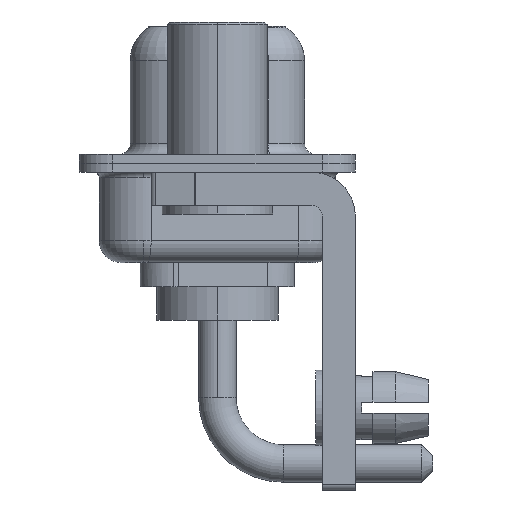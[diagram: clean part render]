
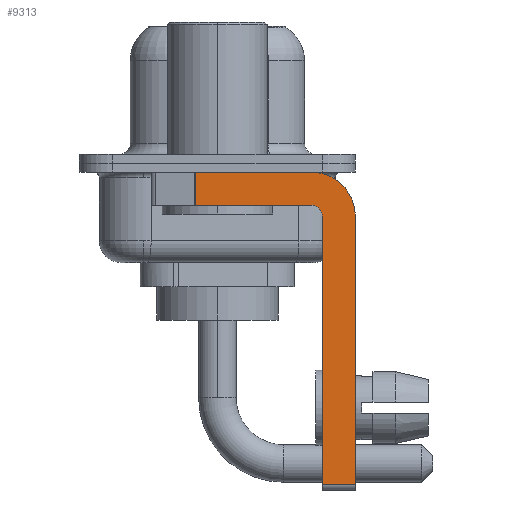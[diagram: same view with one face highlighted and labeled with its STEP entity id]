
A CAD part, left-side view. The second image highlights one B-rep face of the part: STEP entity #9313.
In plain terms, the highlighted planar face has unit normal (-1, 0, 0).
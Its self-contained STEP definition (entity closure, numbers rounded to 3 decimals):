
#875 = CARTESIAN_POINT ( 'NONE',  ( -2.9, -6.25, -14.55 ) ) ;
#929 = CARTESIAN_POINT ( 'NONE',  ( -2.9, -6.25, -2.4 ) ) ;
#1006 = DIRECTION ( 'NONE',  ( 0., -1., 0. ) ) ;
#1123 = EDGE_CURVE ( 'NONE', #10890, #2275, #14505, .T. ) ;
#1128 = VECTOR ( 'NONE', #12689, 1000. ) ;
#1149 = EDGE_CURVE ( 'NONE', #10330, #9300, #10543, .T. ) ;
#1270 = CIRCLE ( 'NONE', #10921, 0.5 ) ;
#1470 = EDGE_CURVE ( 'NONE', #8513, #6060, #1560, .T. ) ;
#1560 = CIRCLE ( 'NONE', #10450, 2. ) ;
#1697 = CARTESIAN_POINT ( 'NONE',  ( -2.9, -4.25, -2.4 ) ) ;
#1864 = DIRECTION ( 'NONE',  ( 0., 0., -1. ) ) ;
#2187 = CARTESIAN_POINT ( 'NONE',  ( -2.9, -4.25, -14.55 ) ) ;
#2262 = CARTESIAN_POINT ( 'NONE',  ( -2.9, -4.25, -2.4 ) ) ;
#2275 = VERTEX_POINT ( 'NONE', #7239 ) ;
#2492 = ORIENTED_EDGE ( 'NONE', *, *, #4163, .T. ) ;
#2978 = VERTEX_POINT ( 'NONE', #14285 ) ;
#2998 = CARTESIAN_POINT ( 'NONE',  ( -2.9, 0.978, -1.9 ) ) ;
#3002 = ORIENTED_EDGE ( 'NONE', *, *, #9882, .F. ) ;
#3699 = CARTESIAN_POINT ( 'NONE',  ( -2.9, -4.25, -1.9 ) ) ;
#4023 = ORIENTED_EDGE ( 'NONE', *, *, #15275, .F. ) ;
#4163 = EDGE_CURVE ( 'NONE', #2978, #2275, #4351, .T. ) ;
#4351 = LINE ( 'NONE', #2998, #1128 ) ;
#4562 = DIRECTION ( 'NONE',  ( 0., 1., 0. ) ) ;
#4587 = VECTOR ( 'NONE', #5769, 1000. ) ;
#4977 = LINE ( 'NONE', #9839, #9176 ) ;
#5038 = VECTOR ( 'NONE', #1006, 1000. ) ;
#5769 = DIRECTION ( 'NONE',  ( 0., 0., -1. ) ) ;
#5777 = CARTESIAN_POINT ( 'NONE',  ( -2.9, -6.25, -2.4 ) ) ;
#5827 = CARTESIAN_POINT ( 'NONE',  ( -2.9, 3., -0.4 ) ) ;
#5926 = DIRECTION ( 'NONE',  ( 0., 0., 1. ) ) ;
#6060 = VERTEX_POINT ( 'NONE', #5777 ) ;
#6126 = DIRECTION ( 'NONE',  ( 0., -1., 0. ) ) ;
#6464 = DIRECTION ( 'NONE',  ( 1., 0., 0. ) ) ;
#6652 = VECTOR ( 'NONE', #6126, 1000. ) ;
#7239 = CARTESIAN_POINT ( 'NONE',  ( -2.9, 0.978, -1.9 ) ) ;
#7953 = DIRECTION ( 'NONE',  ( 0., 0., -1. ) ) ;
#8035 = CARTESIAN_POINT ( 'NONE',  ( -2.9, -4.25, -2.4 ) ) ;
#8040 = EDGE_CURVE ( 'NONE', #6060, #9300, #8169, .T. ) ;
#8117 = DIRECTION ( 'NONE',  ( 1., 0., 0. ) ) ;
#8169 = LINE ( 'NONE', #929, #4587 ) ;
#8501 = EDGE_CURVE ( 'NONE', #2978, #8513, #13051, .T. ) ;
#8513 = VERTEX_POINT ( 'NONE', #9946 ) ;
#8569 = CARTESIAN_POINT ( 'NONE',  ( -2.9, -4.75, -14.55 ) ) ;
#9176 = VECTOR ( 'NONE', #13485, 1000. ) ;
#9300 = VERTEX_POINT ( 'NONE', #875 ) ;
#9313 = ADVANCED_FACE ( 'NONE', ( #10635 ), #10561, .F. ) ;
#9355 = CARTESIAN_POINT ( 'NONE',  ( -2.9, -4.75, -2.4 ) ) ;
#9515 = DIRECTION ( 'NONE',  ( -1., 0., 0. ) ) ;
#9839 = CARTESIAN_POINT ( 'NONE',  ( -2.9, -4.75, -14.8 ) ) ;
#9882 = EDGE_CURVE ( 'NONE', #10330, #15215, #4977, .T. ) ;
#9895 = ORIENTED_EDGE ( 'NONE', *, *, #1149, .T. ) ;
#9927 = AXIS2_PLACEMENT_3D ( 'NONE', #8035, #8117, #7953 ) ;
#9946 = CARTESIAN_POINT ( 'NONE',  ( -2.9, -4.25, -0.4 ) ) ;
#10330 = VERTEX_POINT ( 'NONE', #8569 ) ;
#10450 = AXIS2_PLACEMENT_3D ( 'NONE', #1697, #6464, #1864 ) ;
#10543 = LINE ( 'NONE', #2187, #5038 ) ;
#10561 = PLANE ( 'NONE',  #9927 ) ;
#10635 = FACE_OUTER_BOUND ( 'NONE', #13516, .T. ) ;
#10890 = VERTEX_POINT ( 'NONE', #3699 ) ;
#10921 = AXIS2_PLACEMENT_3D ( 'NONE', #2262, #9515, #5926 ) ;
#11419 = ORIENTED_EDGE ( 'NONE', *, *, #1123, .F. ) ;
#11656 = VECTOR ( 'NONE', #4562, 1000. ) ;
#12427 = ORIENTED_EDGE ( 'NONE', *, *, #1470, .F. ) ;
#12689 = DIRECTION ( 'NONE',  ( 0., 0., -1. ) ) ;
#13026 = ORIENTED_EDGE ( 'NONE', *, *, #8501, .F. ) ;
#13051 = LINE ( 'NONE', #5827, #6652 ) ;
#13485 = DIRECTION ( 'NONE',  ( 0., 0., 1. ) ) ;
#13516 = EDGE_LOOP ( 'NONE', ( #13026, #2492, #11419, #4023, #3002, #9895, #15482, #12427 ) ) ;
#14196 = CARTESIAN_POINT ( 'NONE',  ( -2.9, -4.25, -1.9 ) ) ;
#14285 = CARTESIAN_POINT ( 'NONE',  ( -2.9, 0.978, -0.4 ) ) ;
#14505 = LINE ( 'NONE', #14196, #11656 ) ;
#15215 = VERTEX_POINT ( 'NONE', #9355 ) ;
#15275 = EDGE_CURVE ( 'NONE', #15215, #10890, #1270, .T. ) ;
#15482 = ORIENTED_EDGE ( 'NONE', *, *, #8040, .F. ) ;
